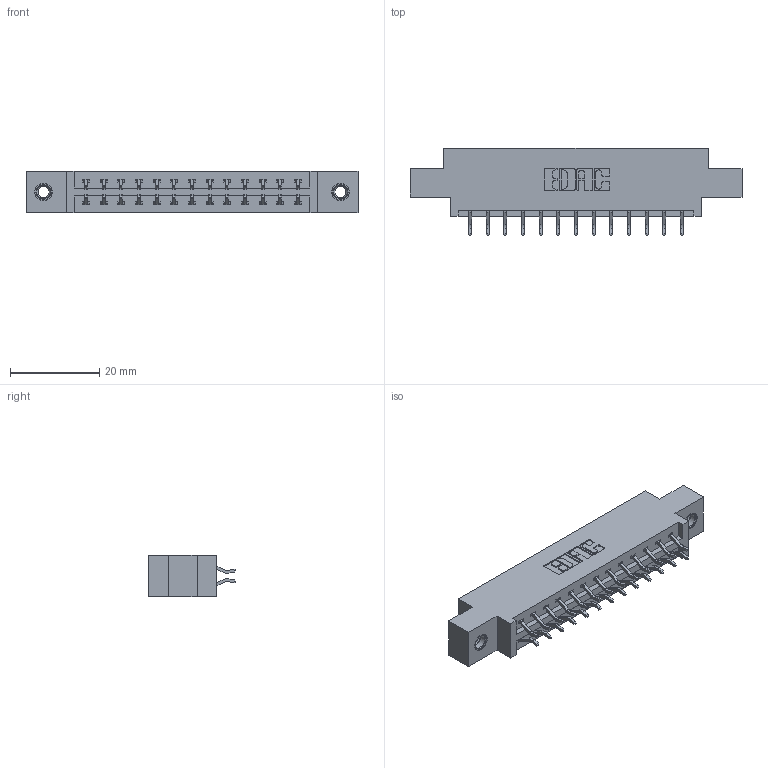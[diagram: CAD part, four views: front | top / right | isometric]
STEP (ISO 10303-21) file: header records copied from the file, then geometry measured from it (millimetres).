
FILE_DESCRIPTION (( 'STEP AP203' ), '1' );
FILE_NAME ('387-026-556-807.STEP', '2019-10-16T20:46:16', ( '' ), ( '' ), 'SwSTEP 2.0', 'SolidWorks 2016', '' );
FILE_SCHEMA (( 'CONFIG_CONTROL_DESIGN' ));
Length unit declared in the file: inch
Products named in the file (4): 387-026-556-807; 337 Part_0.170 Offset - 0.156 Dia-TI; 345-250-001_345-250-005-103; 345-292-001_556 Tail
Assembly tree (29 placements, depth 2):
  387-026-556-807
    337 Part_0.170 Offset - 0.156 Dia-TI
    345-292-001_556 Tail  x26
    345-250-001_345-250-005-103  x2
Bounding box: 74.52 x 19.57 x 9.4 mm (x, y, z)
Volume: 7335.8 mm3; surface area: 8127.8 mm2
Topology: 29 solids, 29 shells, 1738 faces, 5113 edges, 3366 vertices
Faces by surface type: plane 1198, cylinder 524, cone 12, torus 4
Entity records: 15368 total; most frequent: CARTESIAN_POINT 2609, ORIENTED_EDGE 2526, DIRECTION 2293, EDGE_CURVE 1263, LINE 1107, VECTOR 1107, VERTEX_POINT 836, AXIS2_PLACEMENT_3D 593
